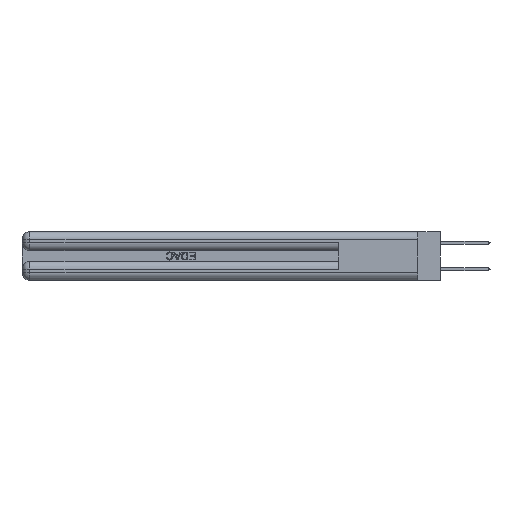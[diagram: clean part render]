
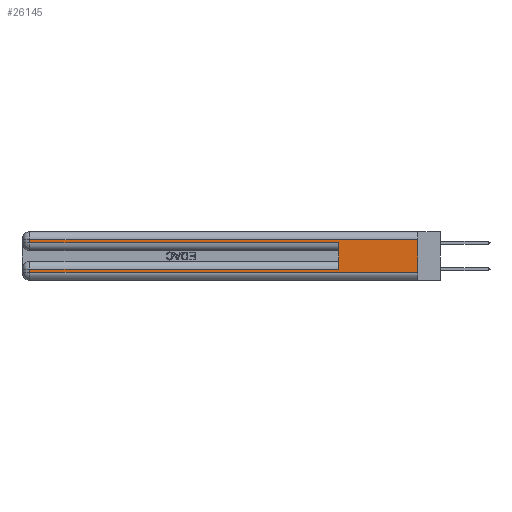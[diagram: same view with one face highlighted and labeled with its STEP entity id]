
A CAD part, left-side view. The second image highlights one B-rep face of the part: STEP entity #26145.
In plain terms, the highlighted planar face has unit normal (-1, 0, 0).
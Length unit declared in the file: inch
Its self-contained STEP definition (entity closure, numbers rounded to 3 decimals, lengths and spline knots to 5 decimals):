
#195 = DIRECTION ( 'NONE',  ( 0., 0., -1. ) ) ;
#1857 = LINE ( 'NONE', #43364, #39576 ) ;
#2092 = CARTESIAN_POINT ( 'NONE',  ( 0., 0., 0.31 ) ) ;
#3058 = ORIENTED_EDGE ( 'NONE', *, *, #41705, .T. ) ;
#5845 = VECTOR ( 'NONE', #41159, 39.37008 ) ;
#6420 = VECTOR ( 'NONE', #25944, 39.37008 ) ;
#6589 = ORIENTED_EDGE ( 'NONE', *, *, #16583, .T. ) ;
#6621 = CARTESIAN_POINT ( 'NONE',  ( 0., 2.94, 0.285 ) ) ;
#7014 = DIRECTION ( 'NONE',  ( 1., 0., 0. ) ) ;
#7758 = ORIENTED_EDGE ( 'NONE', *, *, #40055, .T. ) ;
#8176 = LINE ( 'NONE', #37438, #5845 ) ;
#8968 = VERTEX_POINT ( 'NONE', #48556 ) ;
#10309 = LINE ( 'NONE', #41533, #39181 ) ;
#10710 = CARTESIAN_POINT ( 'NONE',  ( 0., 0., 0.085 ) ) ;
#10802 = DIRECTION ( 'NONE',  ( 0., -1., 0. ) ) ;
#11359 = CARTESIAN_POINT ( 'NONE',  ( 0., 0., 0.285 ) ) ;
#13192 = EDGE_CURVE ( 'NONE', #14161, #39089, #43828, .T. ) ;
#14080 = VECTOR ( 'NONE', #15196, 39.37008 ) ;
#14161 = VERTEX_POINT ( 'NONE', #31506 ) ;
#14918 = EDGE_CURVE ( 'NONE', #22489, #39089, #1857, .T. ) ;
#15196 = DIRECTION ( 'NONE',  ( 0., -1., 0. ) ) ;
#15503 = VERTEX_POINT ( 'NONE', #20769 ) ;
#15955 = VECTOR ( 'NONE', #24787, 39.37008 ) ;
#16577 = LINE ( 'NONE', #10710, #6420 ) ;
#16583 = EDGE_CURVE ( 'NONE', #15503, #36817, #10309, .T. ) ;
#16827 = VECTOR ( 'NONE', #35240, 39.37008 ) ;
#17199 = DIRECTION ( 'NONE',  ( 0., 0., -1. ) ) ;
#17379 = ORIENTED_EDGE ( 'NONE', *, *, #20305, .T. ) ;
#20303 = ORIENTED_EDGE ( 'NONE', *, *, #38839, .F. ) ;
#20305 = EDGE_CURVE ( 'NONE', #24233, #8968, #16577, .T. ) ;
#20769 = CARTESIAN_POINT ( 'NONE',  ( 0., 2.94, 0.31 ) ) ;
#20930 = ORIENTED_EDGE ( 'NONE', *, *, #13192, .T. ) ;
#22489 = VERTEX_POINT ( 'NONE', #36857 ) ;
#24233 = VERTEX_POINT ( 'NONE', #28337 ) ;
#24525 = VERTEX_POINT ( 'NONE', #37322 ) ;
#24787 = DIRECTION ( 'NONE',  ( 0., 1., 0. ) ) ;
#25944 = DIRECTION ( 'NONE',  ( 0., 1., 0. ) ) ;
#25979 = LINE ( 'NONE', #2092, #15955 ) ;
#26145 = ADVANCED_FACE ( 'NONE', ( #30242 ), #29655, .F. ) ;
#27335 = ORIENTED_EDGE ( 'NONE', *, *, #36343, .T. ) ;
#28337 = CARTESIAN_POINT ( 'NONE',  ( 0., 0.6, 0.085 ) ) ;
#28481 = ORIENTED_EDGE ( 'NONE', *, *, #14918, .F. ) ;
#29655 = PLANE ( 'NONE',  #43451 ) ;
#30242 = FACE_OUTER_BOUND ( 'NONE', #44530, .T. ) ;
#31506 = CARTESIAN_POINT ( 'NONE',  ( 0., 2.94, 0.06 ) ) ;
#33387 = CARTESIAN_POINT ( 'NONE',  ( 0., 0., 0.06 ) ) ;
#33425 = DIRECTION ( 'NONE',  ( 0., 0., -1. ) ) ;
#34061 = LINE ( 'NONE', #11359, #14080 ) ;
#35088 = VECTOR ( 'NONE', #10802, 39.37008 ) ;
#35240 = DIRECTION ( 'NONE',  ( 0., 0., -1. ) ) ;
#36343 = EDGE_CURVE ( 'NONE', #8968, #14161, #46693, .T. ) ;
#36817 = VERTEX_POINT ( 'NONE', #6621 ) ;
#36857 = CARTESIAN_POINT ( 'NONE',  ( 0., 0., 0.31 ) ) ;
#37322 = CARTESIAN_POINT ( 'NONE',  ( 0., 0.6, 0.285 ) ) ;
#37438 = CARTESIAN_POINT ( 'NONE',  ( 0., 0.6, 0.145 ) ) ;
#38710 = CARTESIAN_POINT ( 'NONE',  ( 0., 0., 0.06 ) ) ;
#38839 = EDGE_CURVE ( 'NONE', #24233, #24525, #8176, .T. ) ;
#39089 = VERTEX_POINT ( 'NONE', #38710 ) ;
#39181 = VECTOR ( 'NONE', #195, 39.37008 ) ;
#39576 = VECTOR ( 'NONE', #17199, 39.37008 ) ;
#40055 = EDGE_CURVE ( 'NONE', #36817, #24525, #34061, .T. ) ;
#41159 = DIRECTION ( 'NONE',  ( 0., 0., 1. ) ) ;
#41533 = CARTESIAN_POINT ( 'NONE',  ( 0., 2.94, 0.37 ) ) ;
#41705 = EDGE_CURVE ( 'NONE', #22489, #15503, #25979, .T. ) ;
#43364 = CARTESIAN_POINT ( 'NONE',  ( 0., 0., 0.37 ) ) ;
#43451 = AXIS2_PLACEMENT_3D ( 'NONE', #44516, #7014, #33425 ) ;
#43828 = LINE ( 'NONE', #33387, #35088 ) ;
#44516 = CARTESIAN_POINT ( 'NONE',  ( 0., 0., 0.37 ) ) ;
#44530 = EDGE_LOOP ( 'NONE', ( #28481, #3058, #6589, #7758, #20303, #17379, #27335, #20930 ) ) ;
#46322 = CARTESIAN_POINT ( 'NONE',  ( 0., 2.94, 0.37 ) ) ;
#46693 = LINE ( 'NONE', #46322, #16827 ) ;
#48556 = CARTESIAN_POINT ( 'NONE',  ( 0., 2.94, 0.085 ) ) ;
